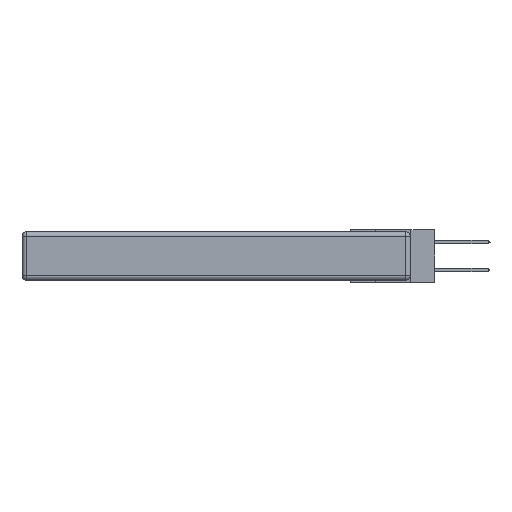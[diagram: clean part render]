
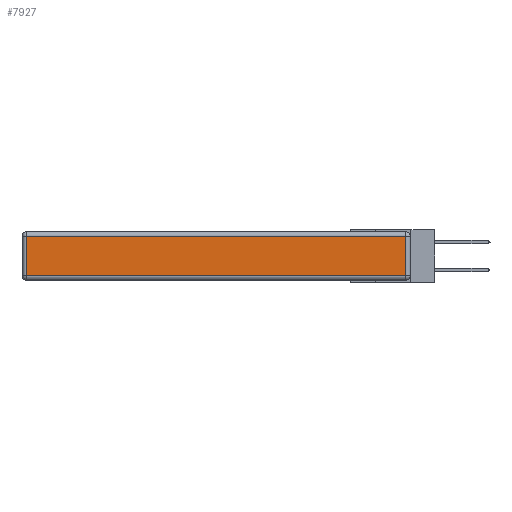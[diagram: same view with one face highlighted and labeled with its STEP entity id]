
A CAD part, left-side view. The second image highlights one B-rep face of the part: STEP entity #7927.
In plain terms, the highlighted planar face has unit normal (-1, 0, 0).
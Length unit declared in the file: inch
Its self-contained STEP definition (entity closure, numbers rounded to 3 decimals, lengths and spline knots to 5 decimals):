
#489 = DIRECTION ( 'NONE',  ( 0., -1., 0. ) ) ;
#1457 = DIRECTION ( 'NONE',  ( 0., 0., 1. ) ) ;
#2603 = EDGE_LOOP ( 'NONE', ( #8125, #20145, #24555, #10167 ) ) ;
#3523 = DIRECTION ( 'NONE',  ( 0., 0., 1. ) ) ;
#4103 = LINE ( 'NONE', #9885, #13599 ) ;
#4479 = VERTEX_POINT ( 'NONE', #11902 ) ;
#5680 = FACE_OUTER_BOUND ( 'NONE', #2603, .T. ) ;
#6718 = EDGE_CURVE ( 'NONE', #24257, #4479, #27325, .T. ) ;
#7927 = ADVANCED_FACE ( 'NONE', ( #5680 ), #16517, .T. ) ;
#8125 = ORIENTED_EDGE ( 'NONE', *, *, #13001, .T. ) ;
#9885 = CARTESIAN_POINT ( 'NONE',  ( 0., 2.75, -0.03 ) ) ;
#10167 = ORIENTED_EDGE ( 'NONE', *, *, #18726, .T. ) ;
#11902 = CARTESIAN_POINT ( 'NONE',  ( 0., 0.03, -0.03 ) ) ;
#13001 = EDGE_CURVE ( 'NONE', #29713, #24257, #31999, .T. ) ;
#13248 = VECTOR ( 'NONE', #489, 39.37008 ) ;
#13599 = VECTOR ( 'NONE', #32792, 39.37008 ) ;
#15100 = VERTEX_POINT ( 'NONE', #18050 ) ;
#16517 = PLANE ( 'NONE',  #22060 ) ;
#18050 = CARTESIAN_POINT ( 'NONE',  ( 0., 2.72, -0.03 ) ) ;
#18726 = EDGE_CURVE ( 'NONE', #15100, #29713, #30674, .T. ) ;
#19931 = EDGE_CURVE ( 'NONE', #4479, #15100, #4103, .T. ) ;
#20145 = ORIENTED_EDGE ( 'NONE', *, *, #6718, .T. ) ;
#20661 = VECTOR ( 'NONE', #20864, 39.37008 ) ;
#20864 = DIRECTION ( 'NONE',  ( 0., 0., -1. ) ) ;
#21446 = DIRECTION ( 'NONE',  ( -1., 0., 0. ) ) ;
#21621 = CARTESIAN_POINT ( 'NONE',  ( 0., 0.03, -0.343 ) ) ;
#22060 = AXIS2_PLACEMENT_3D ( 'NONE', #24255, #21446, #1457 ) ;
#23201 = CARTESIAN_POINT ( 'NONE',  ( 0., 0., -0.313 ) ) ;
#23262 = CARTESIAN_POINT ( 'NONE',  ( 0., 2.72, -0.343 ) ) ;
#24255 = CARTESIAN_POINT ( 'NONE',  ( 0., 0., -0.343 ) ) ;
#24257 = VERTEX_POINT ( 'NONE', #28520 ) ;
#24555 = ORIENTED_EDGE ( 'NONE', *, *, #19931, .T. ) ;
#24902 = VECTOR ( 'NONE', #3523, 39.37008 ) ;
#27325 = LINE ( 'NONE', #21621, #24902 ) ;
#28520 = CARTESIAN_POINT ( 'NONE',  ( 0., 0.03, -0.313 ) ) ;
#29713 = VERTEX_POINT ( 'NONE', #30310 ) ;
#30310 = CARTESIAN_POINT ( 'NONE',  ( 0., 2.72, -0.313 ) ) ;
#30674 = LINE ( 'NONE', #23262, #20661 ) ;
#31999 = LINE ( 'NONE', #23201, #13248 ) ;
#32792 = DIRECTION ( 'NONE',  ( 0., 1., 0. ) ) ;
